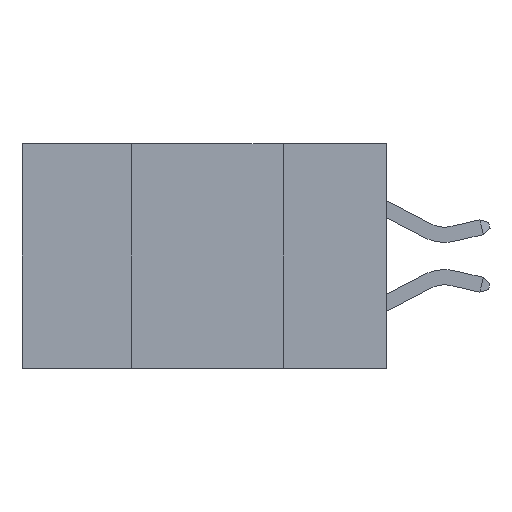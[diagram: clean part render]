
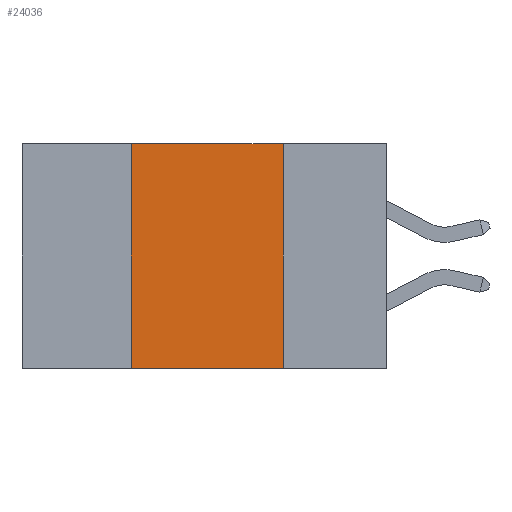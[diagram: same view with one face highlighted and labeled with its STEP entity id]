
A CAD part, left-side view. The second image highlights one B-rep face of the part: STEP entity #24036.
In plain terms, the highlighted planar face has unit normal (-1, 0, 0).
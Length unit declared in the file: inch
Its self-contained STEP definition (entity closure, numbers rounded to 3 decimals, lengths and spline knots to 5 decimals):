
#1772 = CARTESIAN_POINT ( 'NONE',  ( 0., 0.17, 0. ) ) ;
#2464 = EDGE_CURVE ( 'NONE', #9773, #18055, #14346, .T. ) ;
#3489 = CARTESIAN_POINT ( 'NONE',  ( 0., 0.42, 0. ) ) ;
#3957 = LINE ( 'NONE', #17317, #22175 ) ;
#4138 = PLANE ( 'NONE',  #23013 ) ;
#4585 = VECTOR ( 'NONE', #20130, 39.37008 ) ;
#7968 = DIRECTION ( 'NONE',  ( 0., 0., -1. ) ) ;
#8195 = FACE_OUTER_BOUND ( 'NONE', #24117, .T. ) ;
#9773 = VERTEX_POINT ( 'NONE', #20589 ) ;
#10884 = CARTESIAN_POINT ( 'NONE',  ( 0., 0.6, -0.37 ) ) ;
#13323 = VERTEX_POINT ( 'NONE', #24633 ) ;
#13689 = DIRECTION ( 'NONE',  ( 1., 0., 0. ) ) ;
#14005 = ORIENTED_EDGE ( 'NONE', *, *, #17859, .F. ) ;
#14346 = LINE ( 'NONE', #10884, #25540 ) ;
#14931 = ORIENTED_EDGE ( 'NONE', *, *, #20059, .F. ) ;
#17317 = CARTESIAN_POINT ( 'NONE',  ( 0., 0.17, 0. ) ) ;
#17859 = EDGE_CURVE ( 'NONE', #24069, #18055, #3957, .T. ) ;
#18055 = VERTEX_POINT ( 'NONE', #29980 ) ;
#18386 = LINE ( 'NONE', #19734, #30290 ) ;
#19734 = CARTESIAN_POINT ( 'NONE',  ( 0., 0.6, 0. ) ) ;
#20059 = EDGE_CURVE ( 'NONE', #9773, #13323, #29153, .T. ) ;
#20130 = DIRECTION ( 'NONE',  ( 0., 0., 1. ) ) ;
#20589 = CARTESIAN_POINT ( 'NONE',  ( 0., 0.42, -0.37 ) ) ;
#22121 = DIRECTION ( 'NONE',  ( 0., -1., 0. ) ) ;
#22175 = VECTOR ( 'NONE', #7968, 39.37008 ) ;
#23013 = AXIS2_PLACEMENT_3D ( 'NONE', #27963, #13689, #30307 ) ;
#24036 = ADVANCED_FACE ( 'NONE', ( #8195 ), #4138, .F. ) ;
#24069 = VERTEX_POINT ( 'NONE', #1772 ) ;
#24117 = EDGE_LOOP ( 'NONE', ( #14005, #29450, #14931, #25869 ) ) ;
#24633 = CARTESIAN_POINT ( 'NONE',  ( 0., 0.42, 0. ) ) ;
#24824 = DIRECTION ( 'NONE',  ( 0., -1., 0. ) ) ;
#25540 = VECTOR ( 'NONE', #24824, 39.37008 ) ;
#25869 = ORIENTED_EDGE ( 'NONE', *, *, #2464, .T. ) ;
#27963 = CARTESIAN_POINT ( 'NONE',  ( 0., 0.6, 0. ) ) ;
#29126 = EDGE_CURVE ( 'NONE', #13323, #24069, #18386, .T. ) ;
#29153 = LINE ( 'NONE', #3489, #4585 ) ;
#29450 = ORIENTED_EDGE ( 'NONE', *, *, #29126, .F. ) ;
#29980 = CARTESIAN_POINT ( 'NONE',  ( 0., 0.17, -0.37 ) ) ;
#30290 = VECTOR ( 'NONE', #22121, 39.37008 ) ;
#30307 = DIRECTION ( 'NONE',  ( 0., 0., -1. ) ) ;
